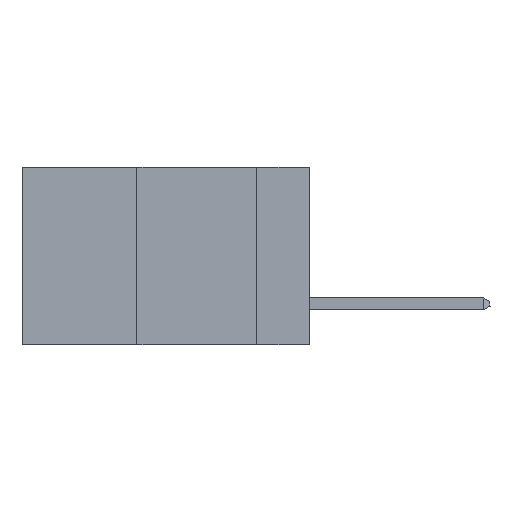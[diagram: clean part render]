
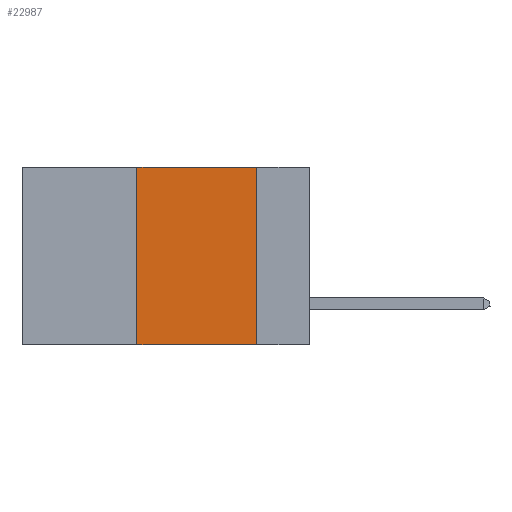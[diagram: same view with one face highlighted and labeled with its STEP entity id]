
A CAD part, left-side view. The second image highlights one B-rep face of the part: STEP entity #22987.
In plain terms, the highlighted planar face has unit normal (-1, 0, 0).
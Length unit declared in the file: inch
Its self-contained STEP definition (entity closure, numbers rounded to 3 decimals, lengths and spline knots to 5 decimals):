
#225 = VERTEX_POINT ( 'NONE', #47192 ) ;
#2673 = LINE ( 'NONE', #29447, #39412 ) ;
#6187 = EDGE_CURVE ( 'NONE', #23372, #20824, #15864, .T. ) ;
#7174 = LINE ( 'NONE', #37522, #35021 ) ;
#9512 = CARTESIAN_POINT ( 'NONE',  ( 0., 0.6, -0.37 ) ) ;
#9742 = LINE ( 'NONE', #9512, #30407 ) ;
#10458 = DIRECTION ( 'NONE',  ( 0., 0., -1. ) ) ;
#12593 = EDGE_CURVE ( 'NONE', #225, #23372, #7174, .T. ) ;
#13337 = DIRECTION ( 'NONE',  ( 0., -1., 0. ) ) ;
#14384 = AXIS2_PLACEMENT_3D ( 'NONE', #35599, #27502, #24019 ) ;
#14687 = CARTESIAN_POINT ( 'NONE',  ( 0., 0.11, 0. ) ) ;
#14701 = VECTOR ( 'NONE', #19823, 39.37008 ) ;
#15864 = LINE ( 'NONE', #33614, #14701 ) ;
#19455 = CARTESIAN_POINT ( 'NONE',  ( 0., 0.36, 0. ) ) ;
#19823 = DIRECTION ( 'NONE',  ( 0., -1., 0. ) ) ;
#20824 = VERTEX_POINT ( 'NONE', #14687 ) ;
#22332 = ORIENTED_EDGE ( 'NONE', *, *, #23242, .F. ) ;
#22987 = ADVANCED_FACE ( 'NONE', ( #34641 ), #31612, .F. ) ;
#23242 = EDGE_CURVE ( 'NONE', #20824, #24190, #2673, .T. ) ;
#23372 = VERTEX_POINT ( 'NONE', #19455 ) ;
#23681 = EDGE_CURVE ( 'NONE', #225, #24190, #9742, .T. ) ;
#24019 = DIRECTION ( 'NONE',  ( 0., 0., -1. ) ) ;
#24190 = VERTEX_POINT ( 'NONE', #39574 ) ;
#27502 = DIRECTION ( 'NONE',  ( 1., 0., 0. ) ) ;
#29447 = CARTESIAN_POINT ( 'NONE',  ( 0., 0.11, 0. ) ) ;
#29613 = ORIENTED_EDGE ( 'NONE', *, *, #6187, .F. ) ;
#30407 = VECTOR ( 'NONE', #13337, 39.37008 ) ;
#31168 = EDGE_LOOP ( 'NONE', ( #22332, #29613, #31508, #47069 ) ) ;
#31508 = ORIENTED_EDGE ( 'NONE', *, *, #12593, .F. ) ;
#31612 = PLANE ( 'NONE',  #14384 ) ;
#33614 = CARTESIAN_POINT ( 'NONE',  ( 0., 0.6, 0. ) ) ;
#34641 = FACE_OUTER_BOUND ( 'NONE', #31168, .T. ) ;
#35021 = VECTOR ( 'NONE', #48933, 39.37008 ) ;
#35599 = CARTESIAN_POINT ( 'NONE',  ( 0., 0.6, 0. ) ) ;
#37522 = CARTESIAN_POINT ( 'NONE',  ( 0., 0.36, 0. ) ) ;
#39412 = VECTOR ( 'NONE', #10458, 39.37008 ) ;
#39574 = CARTESIAN_POINT ( 'NONE',  ( 0., 0.11, -0.37 ) ) ;
#47069 = ORIENTED_EDGE ( 'NONE', *, *, #23681, .T. ) ;
#47192 = CARTESIAN_POINT ( 'NONE',  ( 0., 0.36, -0.37 ) ) ;
#48933 = DIRECTION ( 'NONE',  ( 0., 0., 1. ) ) ;
